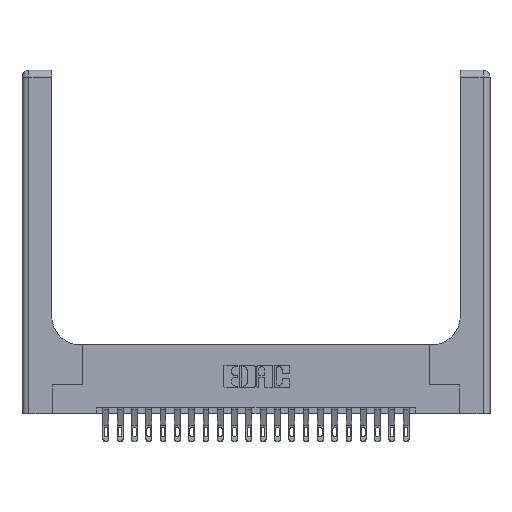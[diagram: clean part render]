
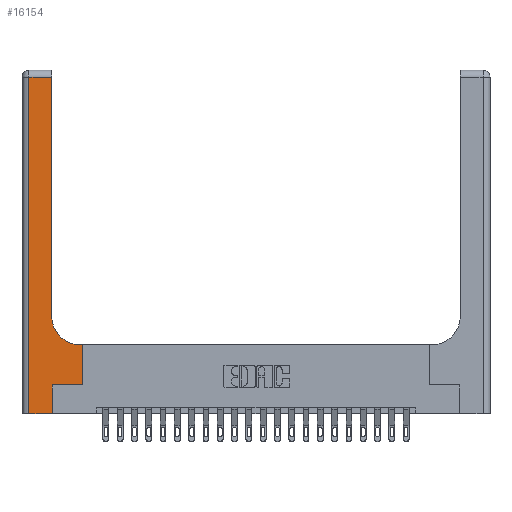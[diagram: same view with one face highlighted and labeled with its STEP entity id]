
A CAD part, top view. The second image highlights one B-rep face of the part: STEP entity #16154.
In plain terms, the highlighted planar face has unit normal (0, 0, 1).
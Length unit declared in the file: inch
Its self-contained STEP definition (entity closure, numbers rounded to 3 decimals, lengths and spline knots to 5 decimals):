
#59 = DIRECTION ( 'NONE',  ( 0., 0., -1. ) ) ;
#104 = VECTOR ( 'NONE', #20793, 39.37008 ) ;
#1097 = CARTESIAN_POINT ( 'NONE',  ( 0.06, 3., 0.37 ) ) ;
#1131 = DIRECTION ( 'NONE',  ( 0., 1., 0. ) ) ;
#1738 = CARTESIAN_POINT ( 'NONE',  ( 0., 0., 0.37 ) ) ;
#1800 = CARTESIAN_POINT ( 'NONE',  ( 0.26, 2.94, 0.37 ) ) ;
#2139 = EDGE_CURVE ( 'NONE', #19540, #19558, #3133, .T. ) ;
#2443 = LINE ( 'NONE', #20234, #2669 ) ;
#2669 = VECTOR ( 'NONE', #15006, 39.37008 ) ;
#2889 = ORIENTED_EDGE ( 'NONE', *, *, #7252, .T. ) ;
#2964 = CARTESIAN_POINT ( 'NONE',  ( 0.528, 0.25, 0.37 ) ) ;
#2975 = VERTEX_POINT ( 'NONE', #1800 ) ;
#3027 = VECTOR ( 'NONE', #7942, 39.37008 ) ;
#3133 = LINE ( 'NONE', #2964, #5642 ) ;
#3358 = CARTESIAN_POINT ( 'NONE',  ( 0.528, 0.25, 0.37 ) ) ;
#3956 = EDGE_CURVE ( 'NONE', #22403, #21876, #9092, .T. ) ;
#4017 = LINE ( 'NONE', #20361, #19013 ) ;
#4461 = ORIENTED_EDGE ( 'NONE', *, *, #9180, .T. ) ;
#4771 = LINE ( 'NONE', #1738, #6428 ) ;
#4808 = CIRCLE ( 'NONE', #8511, 0.25 ) ;
#5568 = AXIS2_PLACEMENT_3D ( 'NONE', #5983, #18168, #6135 ) ;
#5642 = VECTOR ( 'NONE', #13460, 39.37008 ) ;
#5796 = EDGE_CURVE ( 'NONE', #2975, #22403, #8250, .T. ) ;
#5983 = CARTESIAN_POINT ( 'NONE',  ( 0., 3., 0.37 ) ) ;
#6135 = DIRECTION ( 'NONE',  ( -1., 0., 0. ) ) ;
#6428 = VECTOR ( 'NONE', #22378, 39.37008 ) ;
#6728 = DIRECTION ( 'NONE',  ( -1., 0., 0. ) ) ;
#7233 = ORIENTED_EDGE ( 'NONE', *, *, #15862, .T. ) ;
#7252 = EDGE_CURVE ( 'NONE', #16825, #20244, #2443, .T. ) ;
#7942 = DIRECTION ( 'NONE',  ( -1., 0., 0. ) ) ;
#8091 = CARTESIAN_POINT ( 'NONE',  ( 0.265, 0.25, 0.37 ) ) ;
#8250 = LINE ( 'NONE', #19886, #3027 ) ;
#8342 = VECTOR ( 'NONE', #1131, 39.37008 ) ;
#8511 = AXIS2_PLACEMENT_3D ( 'NONE', #15965, #59, #12305 ) ;
#9092 = LINE ( 'NONE', #1097, #21302 ) ;
#9180 = EDGE_CURVE ( 'NONE', #19558, #19364, #4017, .T. ) ;
#9972 = LINE ( 'NONE', #20279, #8342 ) ;
#10297 = CARTESIAN_POINT ( 'NONE',  ( 0.26, 0.85, 0.37 ) ) ;
#12305 = DIRECTION ( 'NONE',  ( 1., 0., 0. ) ) ;
#12465 = VERTEX_POINT ( 'NONE', #10297 ) ;
#13448 = ORIENTED_EDGE ( 'NONE', *, *, #15773, .T. ) ;
#13460 = DIRECTION ( 'NONE',  ( 0., 1., 0. ) ) ;
#14749 = EDGE_CURVE ( 'NONE', #19364, #12465, #4808, .T. ) ;
#15006 = DIRECTION ( 'NONE',  ( 0., 1., 0. ) ) ;
#15246 = ORIENTED_EDGE ( 'NONE', *, *, #2139, .T. ) ;
#15773 = EDGE_CURVE ( 'NONE', #20244, #19540, #17595, .T. ) ;
#15862 = EDGE_CURVE ( 'NONE', #21876, #16825, #4771, .T. ) ;
#15965 = CARTESIAN_POINT ( 'NONE',  ( 0.51, 0.85, 0.37 ) ) ;
#16154 = ADVANCED_FACE ( 'NONE', ( #19208 ), #18018, .F. ) ;
#16182 = ORIENTED_EDGE ( 'NONE', *, *, #18512, .T. ) ;
#16459 = ORIENTED_EDGE ( 'NONE', *, *, #14749, .T. ) ;
#16642 = EDGE_LOOP ( 'NONE', ( #16182, #21878, #16740, #7233, #2889, #13448, #15246, #4461, #16459 ) ) ;
#16740 = ORIENTED_EDGE ( 'NONE', *, *, #3956, .T. ) ;
#16825 = VERTEX_POINT ( 'NONE', #19336 ) ;
#17595 = LINE ( 'NONE', #19076, #104 ) ;
#18018 = PLANE ( 'NONE',  #5568 ) ;
#18168 = DIRECTION ( 'NONE',  ( 0., 0., -1. ) ) ;
#18512 = EDGE_CURVE ( 'NONE', #12465, #2975, #9972, .T. ) ;
#19013 = VECTOR ( 'NONE', #6728, 39.37008 ) ;
#19076 = CARTESIAN_POINT ( 'NONE',  ( 0.265, 0.25, 0.37 ) ) ;
#19208 = FACE_OUTER_BOUND ( 'NONE', #16642, .T. ) ;
#19336 = CARTESIAN_POINT ( 'NONE',  ( 0.265, 0., 0.37 ) ) ;
#19364 = VERTEX_POINT ( 'NONE', #20367 ) ;
#19540 = VERTEX_POINT ( 'NONE', #3358 ) ;
#19558 = VERTEX_POINT ( 'NONE', #22379 ) ;
#19804 = CARTESIAN_POINT ( 'NONE',  ( 0.06, 2.94, 0.37 ) ) ;
#19886 = CARTESIAN_POINT ( 'NONE',  ( 0., 2.94, 0.37 ) ) ;
#20234 = CARTESIAN_POINT ( 'NONE',  ( 0.265, 0., 0.37 ) ) ;
#20244 = VERTEX_POINT ( 'NONE', #8091 ) ;
#20279 = CARTESIAN_POINT ( 'NONE',  ( 0.26, 3., 0.37 ) ) ;
#20361 = CARTESIAN_POINT ( 'NONE',  ( 0.26, 0.6, 0.37 ) ) ;
#20367 = CARTESIAN_POINT ( 'NONE',  ( 0.51, 0.6, 0.37 ) ) ;
#20793 = DIRECTION ( 'NONE',  ( 1., 0., 0. ) ) ;
#21302 = VECTOR ( 'NONE', #22109, 39.37008 ) ;
#21495 = CARTESIAN_POINT ( 'NONE',  ( 0.06, 0., 0.37 ) ) ;
#21876 = VERTEX_POINT ( 'NONE', #21495 ) ;
#21878 = ORIENTED_EDGE ( 'NONE', *, *, #5796, .T. ) ;
#22109 = DIRECTION ( 'NONE',  ( 0., -1., 0. ) ) ;
#22378 = DIRECTION ( 'NONE',  ( 1., 0., 0. ) ) ;
#22379 = CARTESIAN_POINT ( 'NONE',  ( 0.528, 0.6, 0.37 ) ) ;
#22403 = VERTEX_POINT ( 'NONE', #19804 ) ;
